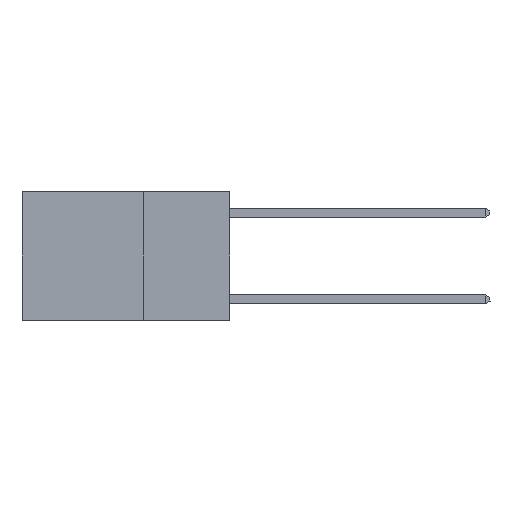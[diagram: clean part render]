
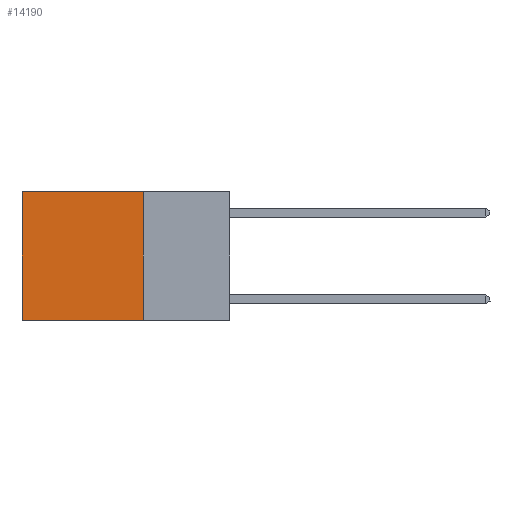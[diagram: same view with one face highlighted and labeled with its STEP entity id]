
A CAD part, left-side view. The second image highlights one B-rep face of the part: STEP entity #14190.
In plain terms, the highlighted planar face has unit normal (-1, 0, 0).
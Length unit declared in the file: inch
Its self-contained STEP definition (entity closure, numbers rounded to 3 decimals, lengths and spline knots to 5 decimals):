
#1290 = LINE ( 'NONE', #4846, #12952 ) ;
#1536 = ORIENTED_EDGE ( 'NONE', *, *, #8075, .F. ) ;
#1817 = DIRECTION ( 'NONE',  ( 0., 1., 0. ) ) ;
#2417 = VERTEX_POINT ( 'NONE', #12609 ) ;
#2520 = CARTESIAN_POINT ( 'NONE',  ( 0.2625, 0.6, 0. ) ) ;
#2649 = VECTOR ( 'NONE', #11575, 39.37008 ) ;
#2702 = CARTESIAN_POINT ( 'NONE',  ( 0.2625, 0.25, 0. ) ) ;
#2729 = DIRECTION ( 'NONE',  ( 1., 0., 0. ) ) ;
#2779 = DIRECTION ( 'NONE',  ( 0., 0., -1. ) ) ;
#3544 = VECTOR ( 'NONE', #1817, 39.37008 ) ;
#3609 = CARTESIAN_POINT ( 'NONE',  ( 0.2625, 0.25, 0. ) ) ;
#4021 = EDGE_CURVE ( 'NONE', #12226, #12406, #13705, .T. ) ;
#4487 = EDGE_LOOP ( 'NONE', ( #12756, #1536, #6825, #10416 ) ) ;
#4846 = CARTESIAN_POINT ( 'NONE',  ( 0.2625, 0.6, 0. ) ) ;
#4972 = CARTESIAN_POINT ( 'NONE',  ( 0.2625, 0.25, 0. ) ) ;
#5571 = FACE_OUTER_BOUND ( 'NONE', #4487, .T. ) ;
#6556 = EDGE_CURVE ( 'NONE', #12226, #9697, #9344, .T. ) ;
#6825 = ORIENTED_EDGE ( 'NONE', *, *, #6556, .F. ) ;
#7859 = VECTOR ( 'NONE', #10755, 39.37008 ) ;
#8075 = EDGE_CURVE ( 'NONE', #9697, #2417, #9227, .T. ) ;
#8706 = EDGE_CURVE ( 'NONE', #12406, #2417, #1290, .T. ) ;
#9227 = LINE ( 'NONE', #12018, #3544 ) ;
#9344 = LINE ( 'NONE', #3609, #2649 ) ;
#9532 = PLANE ( 'NONE',  #13811 ) ;
#9555 = DIRECTION ( 'NONE',  ( 0., 0., -1. ) ) ;
#9697 = VERTEX_POINT ( 'NONE', #10662 ) ;
#10416 = ORIENTED_EDGE ( 'NONE', *, *, #4021, .T. ) ;
#10662 = CARTESIAN_POINT ( 'NONE',  ( 0.2625, 0.25, -0.37 ) ) ;
#10755 = DIRECTION ( 'NONE',  ( 0., 1., 0. ) ) ;
#11575 = DIRECTION ( 'NONE',  ( 0., 0., -1. ) ) ;
#12018 = CARTESIAN_POINT ( 'NONE',  ( 0.2625, 0.25, -0.37 ) ) ;
#12226 = VERTEX_POINT ( 'NONE', #2702 ) ;
#12406 = VERTEX_POINT ( 'NONE', #2520 ) ;
#12609 = CARTESIAN_POINT ( 'NONE',  ( 0.2625, 0.6, -0.37 ) ) ;
#12756 = ORIENTED_EDGE ( 'NONE', *, *, #8706, .T. ) ;
#12952 = VECTOR ( 'NONE', #9555, 39.37008 ) ;
#13705 = LINE ( 'NONE', #4972, #7859 ) ;
#13811 = AXIS2_PLACEMENT_3D ( 'NONE', #13997, #2729, #2779 ) ;
#13997 = CARTESIAN_POINT ( 'NONE',  ( 0.2625, 0.25, 0. ) ) ;
#14190 = ADVANCED_FACE ( 'NONE', ( #5571 ), #9532, .F. ) ;
